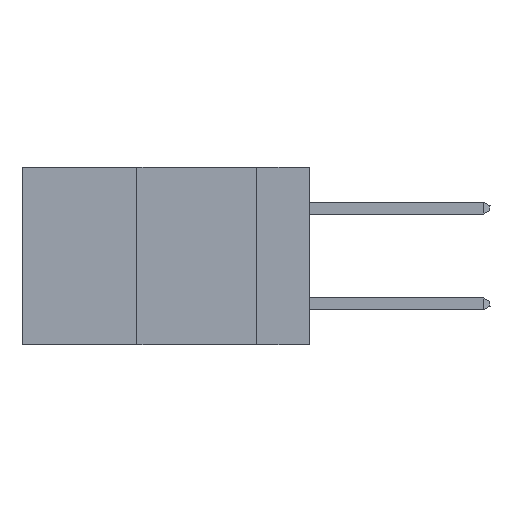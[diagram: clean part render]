
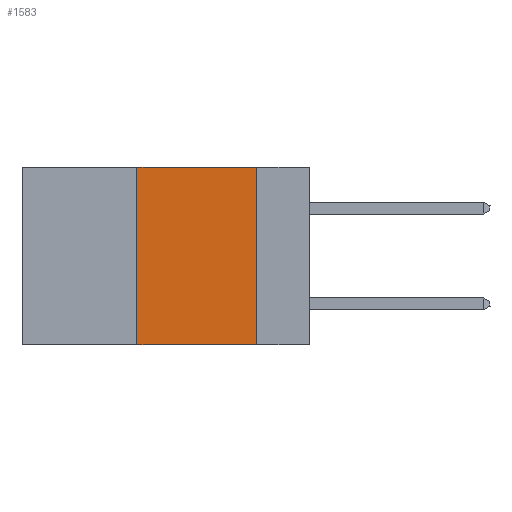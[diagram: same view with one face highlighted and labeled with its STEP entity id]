
A CAD part, left-side view. The second image highlights one B-rep face of the part: STEP entity #1583.
In plain terms, the highlighted planar face has unit normal (-1, 0, 0).
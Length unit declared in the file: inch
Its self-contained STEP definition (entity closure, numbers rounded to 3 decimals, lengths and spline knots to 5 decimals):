
#187 = VERTEX_POINT ( 'NONE', #12291 ) ;
#1583 = ADVANCED_FACE ( 'NONE', ( #16730 ), #5782, .F. ) ;
#1957 = EDGE_CURVE ( 'NONE', #187, #20513, #9709, .T. ) ;
#2191 = VECTOR ( 'NONE', #10883, 39.37008 ) ;
#3420 = DIRECTION ( 'NONE',  ( 0., -1., 0. ) ) ;
#5019 = EDGE_CURVE ( 'NONE', #12794, #18514, #19007, .T. ) ;
#5355 = AXIS2_PLACEMENT_3D ( 'NONE', #10644, #10360, #10127 ) ;
#5782 = PLANE ( 'NONE',  #5355 ) ;
#6296 = VECTOR ( 'NONE', #18275, 39.37008 ) ;
#6479 = LINE ( 'NONE', #16213, #18707 ) ;
#6527 = LINE ( 'NONE', #18701, #2191 ) ;
#7265 = EDGE_CURVE ( 'NONE', #18514, #187, #6479, .T. ) ;
#9326 = CARTESIAN_POINT ( 'NONE',  ( 0., 0.36, -0.37 ) ) ;
#9709 = LINE ( 'NONE', #15576, #17699 ) ;
#10127 = DIRECTION ( 'NONE',  ( 0., 0., -1. ) ) ;
#10360 = DIRECTION ( 'NONE',  ( 1., 0., 0. ) ) ;
#10644 = CARTESIAN_POINT ( 'NONE',  ( 0., 0.6, 0. ) ) ;
#10883 = DIRECTION ( 'NONE',  ( 0., -1., 0. ) ) ;
#12138 = ORIENTED_EDGE ( 'NONE', *, *, #5019, .F. ) ;
#12291 = CARTESIAN_POINT ( 'NONE',  ( 0., 0.11, 0. ) ) ;
#12794 = VERTEX_POINT ( 'NONE', #9326 ) ;
#12986 = ORIENTED_EDGE ( 'NONE', *, *, #13988, .T. ) ;
#13601 = ORIENTED_EDGE ( 'NONE', *, *, #7265, .F. ) ;
#13988 = EDGE_CURVE ( 'NONE', #12794, #20513, #6527, .T. ) ;
#14150 = ORIENTED_EDGE ( 'NONE', *, *, #1957, .F. ) ;
#14296 = CARTESIAN_POINT ( 'NONE',  ( 0., 0.36, 0. ) ) ;
#14953 = DIRECTION ( 'NONE',  ( 0., 0., -1. ) ) ;
#15576 = CARTESIAN_POINT ( 'NONE',  ( 0., 0.11, 0. ) ) ;
#16213 = CARTESIAN_POINT ( 'NONE',  ( 0., 0.6, 0. ) ) ;
#16721 = CARTESIAN_POINT ( 'NONE',  ( 0., 0.36, 0. ) ) ;
#16730 = FACE_OUTER_BOUND ( 'NONE', #18257, .T. ) ;
#17699 = VECTOR ( 'NONE', #14953, 39.37008 ) ;
#17794 = CARTESIAN_POINT ( 'NONE',  ( 0., 0.11, -0.37 ) ) ;
#18257 = EDGE_LOOP ( 'NONE', ( #14150, #13601, #12138, #12986 ) ) ;
#18275 = DIRECTION ( 'NONE',  ( 0., 0., 1. ) ) ;
#18514 = VERTEX_POINT ( 'NONE', #14296 ) ;
#18701 = CARTESIAN_POINT ( 'NONE',  ( 0., 0.6, -0.37 ) ) ;
#18707 = VECTOR ( 'NONE', #3420, 39.37008 ) ;
#19007 = LINE ( 'NONE', #16721, #6296 ) ;
#20513 = VERTEX_POINT ( 'NONE', #17794 ) ;
